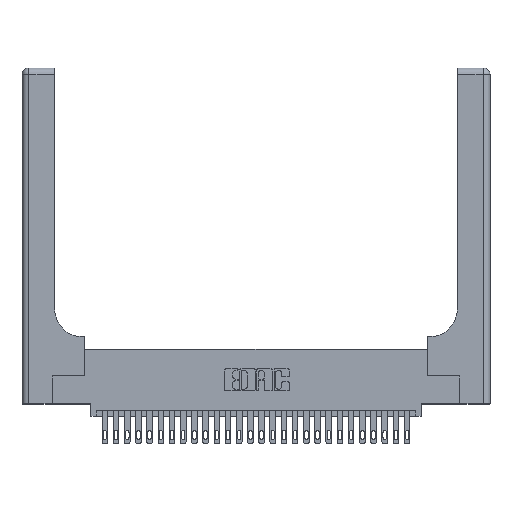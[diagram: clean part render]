
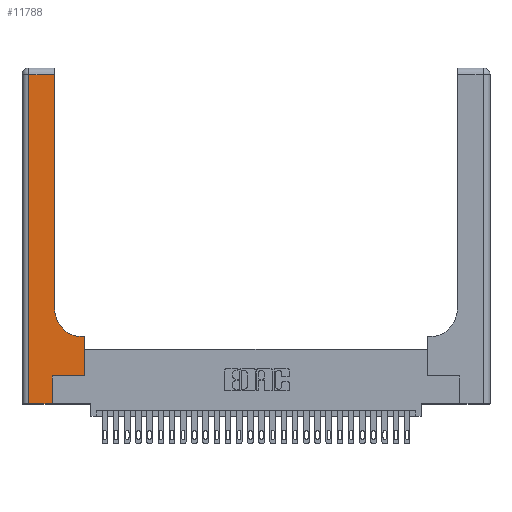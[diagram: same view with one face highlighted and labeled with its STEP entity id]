
A CAD part, top view. The second image highlights one B-rep face of the part: STEP entity #11788.
In plain terms, the highlighted planar face has unit normal (0, 0, 1).
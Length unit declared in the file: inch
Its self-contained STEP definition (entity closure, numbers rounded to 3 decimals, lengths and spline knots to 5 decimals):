
#95 = EDGE_CURVE ( 'NONE', #22155, #8974, #23738, .T. ) ;
#474 = CARTESIAN_POINT ( 'NONE',  ( 0., 2.94, 0.37 ) ) ;
#499 = EDGE_CURVE ( 'NONE', #27292, #23782, #16370, .T. ) ;
#757 = ORIENTED_EDGE ( 'NONE', *, *, #499, .T. ) ;
#1150 = CARTESIAN_POINT ( 'NONE',  ( 0.5585, 0.25, 0.37 ) ) ;
#1438 = EDGE_CURVE ( 'NONE', #23782, #23922, #17281, .T. ) ;
#3267 = CIRCLE ( 'NONE', #4612, 0.25 ) ;
#4491 = CARTESIAN_POINT ( 'NONE',  ( 0.269, 0.25, 0.37 ) ) ;
#4612 = AXIS2_PLACEMENT_3D ( 'NONE', #27487, #22720, #13594 ) ;
#4795 = EDGE_CURVE ( 'NONE', #8974, #25926, #23263, .T. ) ;
#4822 = VECTOR ( 'NONE', #20216, 39.37008 ) ;
#5512 = CARTESIAN_POINT ( 'NONE',  ( 0.5585, 0.25, 0.37 ) ) ;
#5618 = ORIENTED_EDGE ( 'NONE', *, *, #4795, .T. ) ;
#5941 = DIRECTION ( 'NONE',  ( 0., 0., -1. ) ) ;
#6439 = CARTESIAN_POINT ( 'NONE',  ( 0.2915, 0.6, 0.37 ) ) ;
#6606 = EDGE_CURVE ( 'NONE', #7762, #22155, #16151, .T. ) ;
#7172 = LINE ( 'NONE', #19852, #15682 ) ;
#7379 = ORIENTED_EDGE ( 'NONE', *, *, #14980, .T. ) ;
#7521 = DIRECTION ( 'NONE',  ( -1., 0., 0. ) ) ;
#7762 = VERTEX_POINT ( 'NONE', #9967 ) ;
#8974 = VERTEX_POINT ( 'NONE', #1150 ) ;
#9615 = DIRECTION ( 'NONE',  ( 1., 0., 0. ) ) ;
#9967 = CARTESIAN_POINT ( 'NONE',  ( 0.269, 0., 0.37 ) ) ;
#10141 = VECTOR ( 'NONE', #25481, 39.37008 ) ;
#10232 = CARTESIAN_POINT ( 'NONE',  ( 0.2915, 0.85, 0.37 ) ) ;
#10881 = ORIENTED_EDGE ( 'NONE', *, *, #13325, .T. ) ;
#10898 = DIRECTION ( 'NONE',  ( 1., 0., 0. ) ) ;
#11788 = ADVANCED_FACE ( 'NONE', ( #22124 ), #16604, .F. ) ;
#13161 = AXIS2_PLACEMENT_3D ( 'NONE', #21087, #5941, #19447 ) ;
#13239 = DIRECTION ( 'NONE',  ( -1., 0., 0. ) ) ;
#13325 = EDGE_CURVE ( 'NONE', #28459, #27292, #27326, .T. ) ;
#13594 = DIRECTION ( 'NONE',  ( 1., 0., 0. ) ) ;
#14659 = VECTOR ( 'NONE', #9615, 39.37008 ) ;
#14980 = EDGE_CURVE ( 'NONE', #23922, #7762, #7172, .T. ) ;
#15520 = ORIENTED_EDGE ( 'NONE', *, *, #24820, .T. ) ;
#15682 = VECTOR ( 'NONE', #10898, 39.37008 ) ;
#15733 = DIRECTION ( 'NONE',  ( 0., -1., 0. ) ) ;
#16151 = LINE ( 'NONE', #20397, #10141 ) ;
#16370 = LINE ( 'NONE', #474, #23380 ) ;
#16604 = PLANE ( 'NONE',  #13161 ) ;
#16642 = CARTESIAN_POINT ( 'NONE',  ( 0.269, 0.25, 0.37 ) ) ;
#17281 = LINE ( 'NONE', #24356, #23589 ) ;
#19447 = DIRECTION ( 'NONE',  ( -1., 0., 0. ) ) ;
#19852 = CARTESIAN_POINT ( 'NONE',  ( 0., 0., 0.37 ) ) ;
#20216 = DIRECTION ( 'NONE',  ( 0., 1., 0. ) ) ;
#20240 = ORIENTED_EDGE ( 'NONE', *, *, #95, .T. ) ;
#20281 = CARTESIAN_POINT ( 'NONE',  ( 0.5415, 0.6, 0.37 ) ) ;
#20397 = CARTESIAN_POINT ( 'NONE',  ( 0.269, 0., 0.37 ) ) ;
#20842 = EDGE_CURVE ( 'NONE', #22753, #28459, #3267, .T. ) ;
#21005 = ORIENTED_EDGE ( 'NONE', *, *, #1438, .T. ) ;
#21041 = DIRECTION ( 'NONE',  ( 0., 1., 0. ) ) ;
#21087 = CARTESIAN_POINT ( 'NONE',  ( 0., 3., 0.37 ) ) ;
#21924 = EDGE_LOOP ( 'NONE', ( #10881, #757, #21005, #7379, #25356, #20240, #5618, #15520, #23796 ) ) ;
#22124 = FACE_OUTER_BOUND ( 'NONE', #21924, .T. ) ;
#22155 = VERTEX_POINT ( 'NONE', #4491 ) ;
#22366 = CARTESIAN_POINT ( 'NONE',  ( 0.2915, 3., 0.37 ) ) ;
#22419 = CARTESIAN_POINT ( 'NONE',  ( 0.06, 2.94, 0.37 ) ) ;
#22720 = DIRECTION ( 'NONE',  ( 0., 0., -1. ) ) ;
#22753 = VERTEX_POINT ( 'NONE', #20281 ) ;
#23263 = LINE ( 'NONE', #5512, #25005 ) ;
#23380 = VECTOR ( 'NONE', #7521, 39.37008 ) ;
#23589 = VECTOR ( 'NONE', #15733, 39.37008 ) ;
#23738 = LINE ( 'NONE', #16642, #14659 ) ;
#23782 = VERTEX_POINT ( 'NONE', #22419 ) ;
#23796 = ORIENTED_EDGE ( 'NONE', *, *, #20842, .T. ) ;
#23922 = VERTEX_POINT ( 'NONE', #25142 ) ;
#23952 = LINE ( 'NONE', #6439, #24294 ) ;
#24294 = VECTOR ( 'NONE', #13239, 39.37008 ) ;
#24356 = CARTESIAN_POINT ( 'NONE',  ( 0.06, 3., 0.37 ) ) ;
#24820 = EDGE_CURVE ( 'NONE', #25926, #22753, #23952, .T. ) ;
#25005 = VECTOR ( 'NONE', #21041, 39.37008 ) ;
#25142 = CARTESIAN_POINT ( 'NONE',  ( 0.06, 0., 0.37 ) ) ;
#25356 = ORIENTED_EDGE ( 'NONE', *, *, #6606, .T. ) ;
#25481 = DIRECTION ( 'NONE',  ( 0., 1., 0. ) ) ;
#25669 = CARTESIAN_POINT ( 'NONE',  ( 0.5585, 0.6, 0.37 ) ) ;
#25926 = VERTEX_POINT ( 'NONE', #25669 ) ;
#27292 = VERTEX_POINT ( 'NONE', #28892 ) ;
#27326 = LINE ( 'NONE', #22366, #4822 ) ;
#27487 = CARTESIAN_POINT ( 'NONE',  ( 0.5415, 0.85, 0.37 ) ) ;
#28459 = VERTEX_POINT ( 'NONE', #10232 ) ;
#28892 = CARTESIAN_POINT ( 'NONE',  ( 0.2915, 2.94, 0.37 ) ) ;
